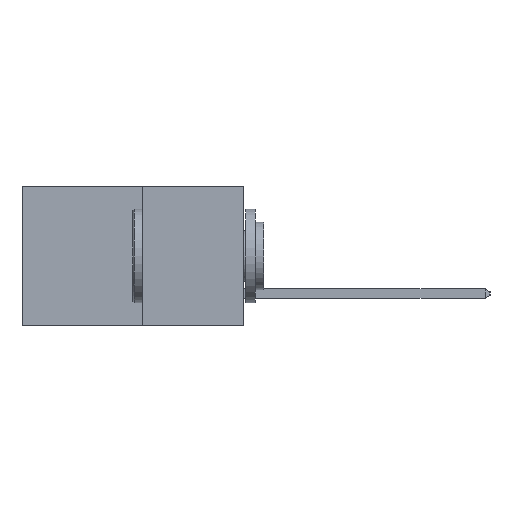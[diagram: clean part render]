
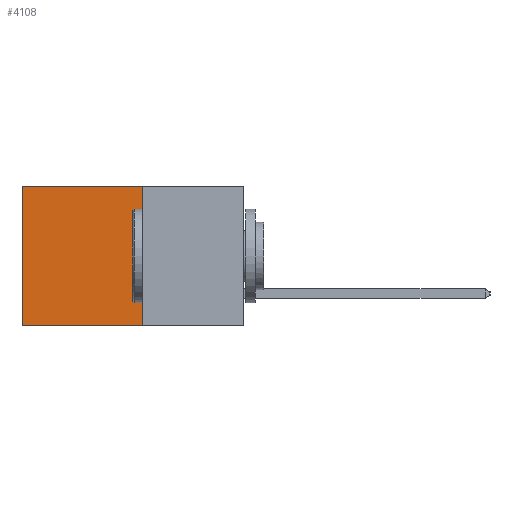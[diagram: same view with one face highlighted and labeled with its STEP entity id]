
A CAD part, left-side view. The second image highlights one B-rep face of the part: STEP entity #4108.
In plain terms, the highlighted planar face has unit normal (-1, 0, 0).
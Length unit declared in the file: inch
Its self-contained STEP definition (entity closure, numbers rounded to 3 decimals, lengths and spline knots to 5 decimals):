
#193 = VERTEX_POINT ( 'NONE', #3703 ) ;
#358 = VERTEX_POINT ( 'NONE', #900 ) ;
#361 = LINE ( 'NONE', #4502, #4426 ) ;
#719 = DIRECTION ( 'NONE',  ( 0., 0., -1. ) ) ;
#900 = CARTESIAN_POINT ( 'NONE',  ( 0.277, 0.27, 0. ) ) ;
#916 = CARTESIAN_POINT ( 'NONE',  ( 0.277, 0.27, -0.37 ) ) ;
#1043 = DIRECTION ( 'NONE',  ( 0., 1., 0. ) ) ;
#1460 = DIRECTION ( 'NONE',  ( 0., 0., -1. ) ) ;
#1488 = DIRECTION ( 'NONE',  ( 1., 0., 0. ) ) ;
#1589 = CARTESIAN_POINT ( 'NONE',  ( 0.277, 0.59, -0.37 ) ) ;
#1889 = VECTOR ( 'NONE', #1043, 39.37008 ) ;
#1898 = VECTOR ( 'NONE', #7277, 39.37008 ) ;
#2759 = CARTESIAN_POINT ( 'NONE',  ( 0.277, 0.27, -0.37 ) ) ;
#3084 = EDGE_LOOP ( 'NONE', ( #3826, #4068, #4392, #4739 ) ) ;
#3419 = FACE_OUTER_BOUND ( 'NONE', #3084, .T. ) ;
#3703 = CARTESIAN_POINT ( 'NONE',  ( 0.277, 0.59, -0.37 ) ) ;
#3826 = ORIENTED_EDGE ( 'NONE', *, *, #8812, .T. ) ;
#3859 = LINE ( 'NONE', #7237, #1898 ) ;
#4068 = ORIENTED_EDGE ( 'NONE', *, *, #5391, .F. ) ;
#4108 = ADVANCED_FACE ( 'NONE', ( #3419 ), #4734, .F. ) ;
#4195 = CARTESIAN_POINT ( 'NONE',  ( 0.277, 0.27, -0.37 ) ) ;
#4226 = VECTOR ( 'NONE', #8119, 39.37008 ) ;
#4392 = ORIENTED_EDGE ( 'NONE', *, *, #6919, .F. ) ;
#4426 = VECTOR ( 'NONE', #719, 39.37008 ) ;
#4502 = CARTESIAN_POINT ( 'NONE',  ( 0.277, 0.27, -0.37 ) ) ;
#4734 = PLANE ( 'NONE',  #8511 ) ;
#4739 = ORIENTED_EDGE ( 'NONE', *, *, #4974, .T. ) ;
#4974 = EDGE_CURVE ( 'NONE', #358, #9305, #3859, .T. ) ;
#5391 = EDGE_CURVE ( 'NONE', #8465, #193, #5810, .T. ) ;
#5810 = LINE ( 'NONE', #916, #1889 ) ;
#6143 = LINE ( 'NONE', #1589, #4226 ) ;
#6919 = EDGE_CURVE ( 'NONE', #358, #8465, #361, .T. ) ;
#7237 = CARTESIAN_POINT ( 'NONE',  ( 0.277, 0.27, 0. ) ) ;
#7277 = DIRECTION ( 'NONE',  ( 0., 1., 0. ) ) ;
#8119 = DIRECTION ( 'NONE',  ( 0., 0., -1. ) ) ;
#8465 = VERTEX_POINT ( 'NONE', #2759 ) ;
#8511 = AXIS2_PLACEMENT_3D ( 'NONE', #4195, #1488, #1460 ) ;
#8680 = CARTESIAN_POINT ( 'NONE',  ( 0.277, 0.59, 0. ) ) ;
#8812 = EDGE_CURVE ( 'NONE', #9305, #193, #6143, .T. ) ;
#9305 = VERTEX_POINT ( 'NONE', #8680 ) ;
